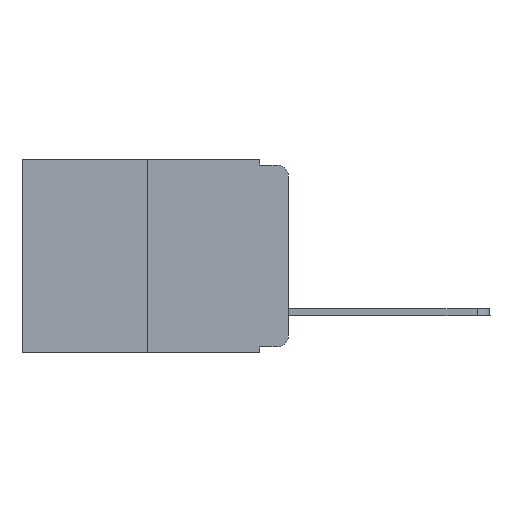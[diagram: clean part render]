
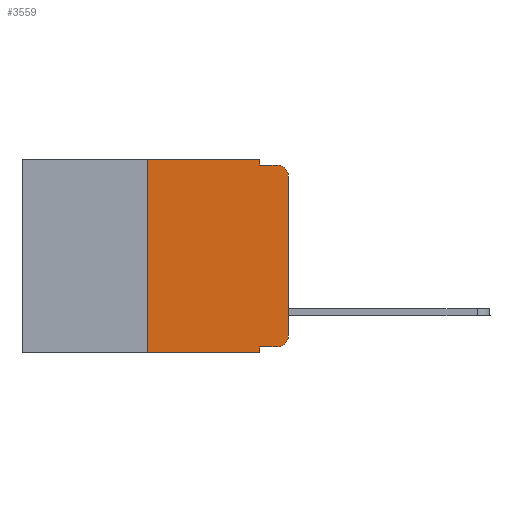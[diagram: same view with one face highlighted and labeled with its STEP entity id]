
A CAD part, left-side view. The second image highlights one B-rep face of the part: STEP entity #3559.
In plain terms, the highlighted planar face has unit normal (-1, 0, 0).
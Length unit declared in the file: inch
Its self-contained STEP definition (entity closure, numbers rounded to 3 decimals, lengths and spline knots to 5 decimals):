
#57 = DIRECTION ( 'NONE',  ( 0., 0., -1. ) ) ;
#93 = CIRCLE ( 'NONE', #10501, 0.02 ) ;
#124 = VECTOR ( 'NONE', #12342, 39.37008 ) ;
#134 = VERTEX_POINT ( 'NONE', #14790 ) ;
#341 = DIRECTION ( 'NONE',  ( 0., 0., 1. ) ) ;
#378 = DIRECTION ( 'NONE',  ( 0., 0., -1. ) ) ;
#435 = ORIENTED_EDGE ( 'NONE', *, *, #3504, .F. ) ;
#745 = PLANE ( 'NONE',  #1589 ) ;
#916 = DIRECTION ( 'NONE',  ( 0., -1., 0. ) ) ;
#982 = DIRECTION ( 'NONE',  ( 0., 0., -1. ) ) ;
#1301 = LINE ( 'NONE', #9126, #15358 ) ;
#1589 = AXIS2_PLACEMENT_3D ( 'NONE', #13251, #7611, #17091 ) ;
#1822 = EDGE_CURVE ( 'NONE', #7661, #6893, #17108, .T. ) ;
#2038 = DIRECTION ( 'NONE',  ( 0., -1., 0. ) ) ;
#2755 = CARTESIAN_POINT ( 'NONE',  ( 0., 0.051, -0.343 ) ) ;
#2790 = VECTOR ( 'NONE', #341, 39.37008 ) ;
#2818 = LINE ( 'NONE', #10136, #9424 ) ;
#3090 = ORIENTED_EDGE ( 'NONE', *, *, #6882, .F. ) ;
#3104 = LINE ( 'NONE', #4124, #17551 ) ;
#3271 = EDGE_CURVE ( 'NONE', #7661, #5497, #14936, .T. ) ;
#3504 = EDGE_CURVE ( 'NONE', #14199, #6893, #1301, .T. ) ;
#3559 = ADVANCED_FACE ( 'NONE', ( #11510 ), #745, .F. ) ;
#3605 = VERTEX_POINT ( 'NONE', #7345 ) ;
#3637 = ORIENTED_EDGE ( 'NONE', *, *, #17306, .T. ) ;
#4124 = CARTESIAN_POINT ( 'NONE',  ( 0., 0.051, 0. ) ) ;
#4210 = ORIENTED_EDGE ( 'NONE', *, *, #6600, .T. ) ;
#4216 = VERTEX_POINT ( 'NONE', #4859 ) ;
#4698 = ORIENTED_EDGE ( 'NONE', *, *, #10592, .F. ) ;
#4859 = CARTESIAN_POINT ( 'NONE',  ( 0., 0., -0.313 ) ) ;
#5497 = VERTEX_POINT ( 'NONE', #13447 ) ;
#5855 = CIRCLE ( 'NONE', #16256, 0.02 ) ;
#5979 = DIRECTION ( 'NONE',  ( 0., -1., 0. ) ) ;
#6568 = EDGE_LOOP ( 'NONE', ( #4210, #3637, #14114, #3090, #4698, #10877, #7668, #435, #12895, #13448 ) ) ;
#6589 = VERTEX_POINT ( 'NONE', #9589 ) ;
#6600 = EDGE_CURVE ( 'NONE', #4216, #12256, #15461, .T. ) ;
#6657 = VERTEX_POINT ( 'NONE', #13293 ) ;
#6882 = EDGE_CURVE ( 'NONE', #3605, #6657, #3104, .T. ) ;
#6893 = VERTEX_POINT ( 'NONE', #2755 ) ;
#7345 = CARTESIAN_POINT ( 'NONE',  ( 0., 0.051, 0. ) ) ;
#7611 = DIRECTION ( 'NONE',  ( 1., 0., 0. ) ) ;
#7661 = VERTEX_POINT ( 'NONE', #9706 ) ;
#7668 = ORIENTED_EDGE ( 'NONE', *, *, #1822, .T. ) ;
#7673 = CARTESIAN_POINT ( 'NONE',  ( 0., 0.473, 0. ) ) ;
#7820 = DIRECTION ( 'NONE',  ( -1., 0., 0. ) ) ;
#8151 = LINE ( 'NONE', #7673, #13254 ) ;
#8348 = DIRECTION ( 'NONE',  ( -1., 0., 0. ) ) ;
#8550 = EDGE_CURVE ( 'NONE', #6657, #6589, #14213, .T. ) ;
#9025 = CARTESIAN_POINT ( 'NONE',  ( 0., 0.473, -0.343 ) ) ;
#9126 = CARTESIAN_POINT ( 'NONE',  ( 0., 0.051, 0. ) ) ;
#9424 = VECTOR ( 'NONE', #2038, 39.37008 ) ;
#9508 = EDGE_CURVE ( 'NONE', #134, #4216, #93, .T. ) ;
#9589 = CARTESIAN_POINT ( 'NONE',  ( 0., 0.02, -0.01 ) ) ;
#9706 = CARTESIAN_POINT ( 'NONE',  ( 0., 0.25, -0.343 ) ) ;
#9723 = VECTOR ( 'NONE', #5979, 39.37008 ) ;
#9781 = CARTESIAN_POINT ( 'NONE',  ( 0., 0.051, -0.333 ) ) ;
#10136 = CARTESIAN_POINT ( 'NONE',  ( 0., 0.051, -0.333 ) ) ;
#10501 = AXIS2_PLACEMENT_3D ( 'NONE', #11084, #8348, #378 ) ;
#10592 = EDGE_CURVE ( 'NONE', #5497, #3605, #8151, .T. ) ;
#10710 = EDGE_CURVE ( 'NONE', #14199, #134, #2818, .T. ) ;
#10783 = CARTESIAN_POINT ( 'NONE',  ( 0., 0., 0. ) ) ;
#10877 = ORIENTED_EDGE ( 'NONE', *, *, #3271, .F. ) ;
#11084 = CARTESIAN_POINT ( 'NONE',  ( 0., 0.02, -0.313 ) ) ;
#11510 = FACE_OUTER_BOUND ( 'NONE', #6568, .T. ) ;
#11797 = VECTOR ( 'NONE', #13108, 39.37008 ) ;
#12256 = VERTEX_POINT ( 'NONE', #15844 ) ;
#12342 = DIRECTION ( 'NONE',  ( 0., 0., 1. ) ) ;
#12895 = ORIENTED_EDGE ( 'NONE', *, *, #10710, .T. ) ;
#13108 = DIRECTION ( 'NONE',  ( 0., -1., 0. ) ) ;
#13251 = CARTESIAN_POINT ( 'NONE',  ( 0., 0.473, 0. ) ) ;
#13254 = VECTOR ( 'NONE', #916, 39.37008 ) ;
#13293 = CARTESIAN_POINT ( 'NONE',  ( 0., 0.051, -0.01 ) ) ;
#13447 = CARTESIAN_POINT ( 'NONE',  ( 0., 0.25, 0. ) ) ;
#13448 = ORIENTED_EDGE ( 'NONE', *, *, #9508, .T. ) ;
#14114 = ORIENTED_EDGE ( 'NONE', *, *, #8550, .F. ) ;
#14199 = VERTEX_POINT ( 'NONE', #9781 ) ;
#14213 = LINE ( 'NONE', #15141, #9723 ) ;
#14790 = CARTESIAN_POINT ( 'NONE',  ( 0., 0.02, -0.333 ) ) ;
#14936 = LINE ( 'NONE', #16566, #2790 ) ;
#15141 = CARTESIAN_POINT ( 'NONE',  ( 0., 0.051, -0.01 ) ) ;
#15358 = VECTOR ( 'NONE', #982, 39.37008 ) ;
#15461 = LINE ( 'NONE', #10783, #124 ) ;
#15844 = CARTESIAN_POINT ( 'NONE',  ( 0., 0., -0.03 ) ) ;
#16256 = AXIS2_PLACEMENT_3D ( 'NONE', #17346, #7820, #17238 ) ;
#16566 = CARTESIAN_POINT ( 'NONE',  ( 0., 0.25, 0. ) ) ;
#17091 = DIRECTION ( 'NONE',  ( 0., 0., -1. ) ) ;
#17108 = LINE ( 'NONE', #9025, #11797 ) ;
#17238 = DIRECTION ( 'NONE',  ( 0., 0., -1. ) ) ;
#17306 = EDGE_CURVE ( 'NONE', #12256, #6589, #5855, .T. ) ;
#17346 = CARTESIAN_POINT ( 'NONE',  ( 0., 0.02, -0.03 ) ) ;
#17551 = VECTOR ( 'NONE', #57, 39.37008 ) ;
